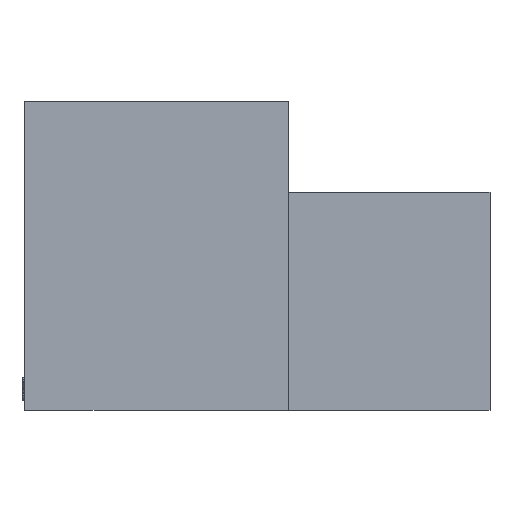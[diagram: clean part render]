
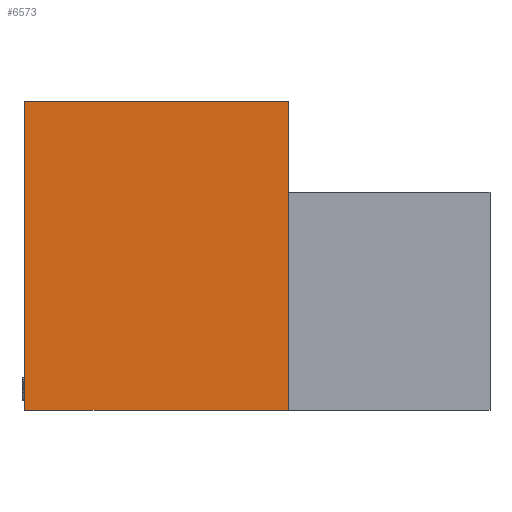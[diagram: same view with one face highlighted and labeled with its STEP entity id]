
A CAD part, left-side view. The second image highlights one B-rep face of the part: STEP entity #6573.
In plain terms, the highlighted planar face has unit normal (-1, 0, 0).
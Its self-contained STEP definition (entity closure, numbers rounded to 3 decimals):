
#449 = LINE ( 'NONE', #8366, #17408 ) ;
#1655 = CARTESIAN_POINT ( 'NONE',  ( 0., 11.506, 0. ) ) ;
#2466 = DIRECTION ( 'NONE',  ( 0., 0., -1. ) ) ;
#2910 = VERTEX_POINT ( 'NONE', #8086 ) ;
#3603 = LINE ( 'NONE', #1655, #9085 ) ;
#3634 = LINE ( 'NONE', #15489, #9348 ) ;
#4675 = ORIENTED_EDGE ( 'NONE', *, *, #18699, .F. ) ;
#4713 = VECTOR ( 'NONE', #2466, 1000. ) ;
#4756 = CARTESIAN_POINT ( 'NONE',  ( 0., 0., 0. ) ) ;
#4999 = EDGE_CURVE ( 'NONE', #12259, #15504, #3634, .T. ) ;
#5033 = CARTESIAN_POINT ( 'NONE',  ( 0., 11.506, -13.487 ) ) ;
#5361 = DIRECTION ( 'NONE',  ( 0., 0., -1. ) ) ;
#5502 = CARTESIAN_POINT ( 'NONE',  ( 0., 0., 0. ) ) ;
#6006 = DIRECTION ( 'NONE',  ( 0., 1., 0. ) ) ;
#6573 = ADVANCED_FACE ( 'NONE', ( #9521 ), #11602, .F. ) ;
#7920 = LINE ( 'NONE', #17096, #4713 ) ;
#8086 = CARTESIAN_POINT ( 'NONE',  ( 0., 11.506, 0. ) ) ;
#8366 = CARTESIAN_POINT ( 'NONE',  ( 0., 11.506, -13.487 ) ) ;
#9085 = VECTOR ( 'NONE', #11264, 1000. ) ;
#9348 = VECTOR ( 'NONE', #6006, 1000. ) ;
#9521 = FACE_OUTER_BOUND ( 'NONE', #18024, .T. ) ;
#9537 = AXIS2_PLACEMENT_3D ( 'NONE', #5502, #14912, #5361 ) ;
#9867 = CARTESIAN_POINT ( 'NONE',  ( 0., 0., -13.487 ) ) ;
#9961 = VERTEX_POINT ( 'NONE', #4756 ) ;
#11264 = DIRECTION ( 'NONE',  ( 0., -1., 0. ) ) ;
#11602 = PLANE ( 'NONE',  #9537 ) ;
#12259 = VERTEX_POINT ( 'NONE', #9867 ) ;
#14289 = EDGE_CURVE ( 'NONE', #2910, #9961, #3603, .T. ) ;
#14735 = DIRECTION ( 'NONE',  ( 0., 0., 1. ) ) ;
#14881 = ORIENTED_EDGE ( 'NONE', *, *, #14289, .F. ) ;
#14912 = DIRECTION ( 'NONE',  ( 1., 0., 0. ) ) ;
#15489 = CARTESIAN_POINT ( 'NONE',  ( 0., -8.814, -13.487 ) ) ;
#15504 = VERTEX_POINT ( 'NONE', #5033 ) ;
#17096 = CARTESIAN_POINT ( 'NONE',  ( 0., 0., 0. ) ) ;
#17408 = VECTOR ( 'NONE', #14735, 1000. ) ;
#17935 = ORIENTED_EDGE ( 'NONE', *, *, #19015, .F. ) ;
#18024 = EDGE_LOOP ( 'NONE', ( #18195, #17935, #14881, #4675 ) ) ;
#18195 = ORIENTED_EDGE ( 'NONE', *, *, #4999, .F. ) ;
#18699 = EDGE_CURVE ( 'NONE', #15504, #2910, #449, .T. ) ;
#19015 = EDGE_CURVE ( 'NONE', #9961, #12259, #7920, .T. ) ;
